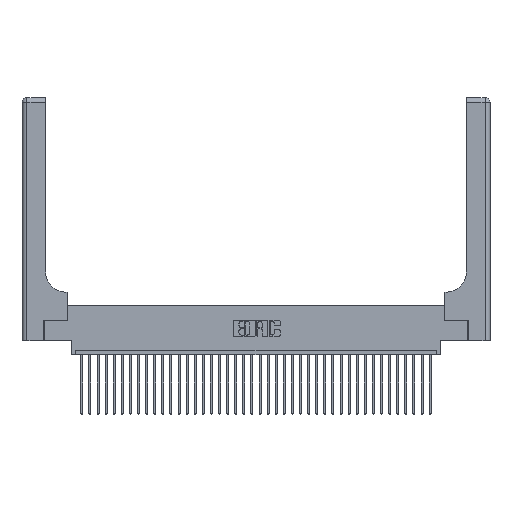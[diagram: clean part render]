
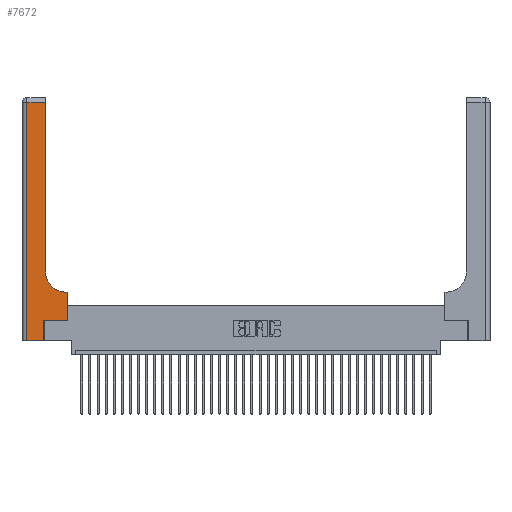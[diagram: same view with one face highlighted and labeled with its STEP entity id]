
A CAD part, top view. The second image highlights one B-rep face of the part: STEP entity #7672.
In plain terms, the highlighted planar face has unit normal (0, 0, 1).
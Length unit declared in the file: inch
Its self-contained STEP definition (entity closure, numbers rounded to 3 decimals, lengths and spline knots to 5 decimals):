
#181 = CARTESIAN_POINT ( 'NONE',  ( 0.06, 2.94, 0.37 ) ) ;
#192 = VECTOR ( 'NONE', #19215, 39.37008 ) ;
#1303 = EDGE_LOOP ( 'NONE', ( #9990, #26657, #36289, #34651, #2468, #13953, #29189, #34596, #16670 ) ) ;
#1619 = VERTEX_POINT ( 'NONE', #4120 ) ;
#2033 = LINE ( 'NONE', #27874, #29707 ) ;
#2147 = DIRECTION ( 'NONE',  ( 0., 1., 0. ) ) ;
#2468 = ORIENTED_EDGE ( 'NONE', *, *, #8235, .T. ) ;
#3025 = EDGE_CURVE ( 'NONE', #37259, #1619, #13595, .T. ) ;
#3908 = EDGE_CURVE ( 'NONE', #1619, #22263, #19573, .T. ) ;
#4120 = CARTESIAN_POINT ( 'NONE',  ( 0.2915, 2.94, 0.37 ) ) ;
#4953 = CARTESIAN_POINT ( 'NONE',  ( 0.2915, 3., 0.37 ) ) ;
#5163 = CARTESIAN_POINT ( 'NONE',  ( 0.269, 0., 0.37 ) ) ;
#5848 = LINE ( 'NONE', #13549, #23875 ) ;
#7220 = DIRECTION ( 'NONE',  ( 0., 0., -1. ) ) ;
#7672 = ADVANCED_FACE ( 'NONE', ( #27695 ), #14699, .F. ) ;
#8235 = EDGE_CURVE ( 'NONE', #13135, #26112, #12929, .T. ) ;
#8402 = DIRECTION ( 'NONE',  ( 0., -1., 0. ) ) ;
#9990 = ORIENTED_EDGE ( 'NONE', *, *, #3025, .T. ) ;
#11345 = CARTESIAN_POINT ( 'NONE',  ( 0.2915, 0.6, 0.37 ) ) ;
#12192 = VERTEX_POINT ( 'NONE', #15456 ) ;
#12335 = EDGE_CURVE ( 'NONE', #26112, #31695, #2033, .T. ) ;
#12716 = AXIS2_PLACEMENT_3D ( 'NONE', #29009, #35064, #32007 ) ;
#12929 = LINE ( 'NONE', #14194, #36002 ) ;
#13042 = CARTESIAN_POINT ( 'NONE',  ( 0.5585, 0.6, 0.37 ) ) ;
#13060 = CARTESIAN_POINT ( 'NONE',  ( 0.5585, 0.25, 0.37 ) ) ;
#13124 = EDGE_CURVE ( 'NONE', #15161, #13135, #32438, .T. ) ;
#13135 = VERTEX_POINT ( 'NONE', #5163 ) ;
#13549 = CARTESIAN_POINT ( 'NONE',  ( 0.06, 3., 0.37 ) ) ;
#13595 = LINE ( 'NONE', #4953, #34386 ) ;
#13953 = ORIENTED_EDGE ( 'NONE', *, *, #12335, .T. ) ;
#14194 = CARTESIAN_POINT ( 'NONE',  ( 0.269, 0., 0.37 ) ) ;
#14699 = PLANE ( 'NONE',  #12716 ) ;
#15161 = VERTEX_POINT ( 'NONE', #28508 ) ;
#15456 = CARTESIAN_POINT ( 'NONE',  ( 0.5415, 0.6, 0.37 ) ) ;
#16670 = ORIENTED_EDGE ( 'NONE', *, *, #18581, .T. ) ;
#16906 = CARTESIAN_POINT ( 'NONE',  ( 0., 2.94, 0.37 ) ) ;
#18581 = EDGE_CURVE ( 'NONE', #12192, #37259, #32256, .T. ) ;
#18683 = EDGE_CURVE ( 'NONE', #31695, #27045, #18889, .T. ) ;
#18889 = LINE ( 'NONE', #34549, #24906 ) ;
#19215 = DIRECTION ( 'NONE',  ( -1., 0., 0. ) ) ;
#19573 = LINE ( 'NONE', #16906, #192 ) ;
#20015 = DIRECTION ( 'NONE',  ( 1., 0., 0. ) ) ;
#22263 = VERTEX_POINT ( 'NONE', #181 ) ;
#22722 = DIRECTION ( 'NONE',  ( 0., 1., 0. ) ) ;
#22833 = DIRECTION ( 'NONE',  ( -1., 0., 0. ) ) ;
#23215 = VECTOR ( 'NONE', #31882, 39.37008 ) ;
#23875 = VECTOR ( 'NONE', #8402, 39.37008 ) ;
#24906 = VECTOR ( 'NONE', #34053, 39.37008 ) ;
#26112 = VERTEX_POINT ( 'NONE', #35473 ) ;
#26657 = ORIENTED_EDGE ( 'NONE', *, *, #3908, .T. ) ;
#27045 = VERTEX_POINT ( 'NONE', #13042 ) ;
#27536 = VECTOR ( 'NONE', #22833, 39.37008 ) ;
#27695 = FACE_OUTER_BOUND ( 'NONE', #1303, .T. ) ;
#27874 = CARTESIAN_POINT ( 'NONE',  ( 0.269, 0.25, 0.37 ) ) ;
#27980 = LINE ( 'NONE', #11345, #27536 ) ;
#28508 = CARTESIAN_POINT ( 'NONE',  ( 0.06, 0., 0.37 ) ) ;
#29009 = CARTESIAN_POINT ( 'NONE',  ( 0., 3., 0.37 ) ) ;
#29189 = ORIENTED_EDGE ( 'NONE', *, *, #18683, .T. ) ;
#29235 = AXIS2_PLACEMENT_3D ( 'NONE', #33802, #7220, #36596 ) ;
#29707 = VECTOR ( 'NONE', #20015, 39.37008 ) ;
#30590 = EDGE_CURVE ( 'NONE', #22263, #15161, #5848, .T. ) ;
#30640 = EDGE_CURVE ( 'NONE', #27045, #12192, #27980, .T. ) ;
#31695 = VERTEX_POINT ( 'NONE', #13060 ) ;
#31882 = DIRECTION ( 'NONE',  ( 1., 0., 0. ) ) ;
#32007 = DIRECTION ( 'NONE',  ( -1., 0., 0. ) ) ;
#32256 = CIRCLE ( 'NONE', #29235, 0.25 ) ;
#32438 = LINE ( 'NONE', #34346, #23215 ) ;
#33802 = CARTESIAN_POINT ( 'NONE',  ( 0.5415, 0.85, 0.37 ) ) ;
#34053 = DIRECTION ( 'NONE',  ( 0., 1., 0. ) ) ;
#34205 = CARTESIAN_POINT ( 'NONE',  ( 0.2915, 0.85, 0.37 ) ) ;
#34346 = CARTESIAN_POINT ( 'NONE',  ( 0., 0., 0.37 ) ) ;
#34386 = VECTOR ( 'NONE', #2147, 39.37008 ) ;
#34549 = CARTESIAN_POINT ( 'NONE',  ( 0.5585, 0.25, 0.37 ) ) ;
#34596 = ORIENTED_EDGE ( 'NONE', *, *, #30640, .T. ) ;
#34651 = ORIENTED_EDGE ( 'NONE', *, *, #13124, .T. ) ;
#35064 = DIRECTION ( 'NONE',  ( 0., 0., -1. ) ) ;
#35473 = CARTESIAN_POINT ( 'NONE',  ( 0.269, 0.25, 0.37 ) ) ;
#36002 = VECTOR ( 'NONE', #22722, 39.37008 ) ;
#36289 = ORIENTED_EDGE ( 'NONE', *, *, #30590, .T. ) ;
#36596 = DIRECTION ( 'NONE',  ( 1., 0., 0. ) ) ;
#37259 = VERTEX_POINT ( 'NONE', #34205 ) ;
